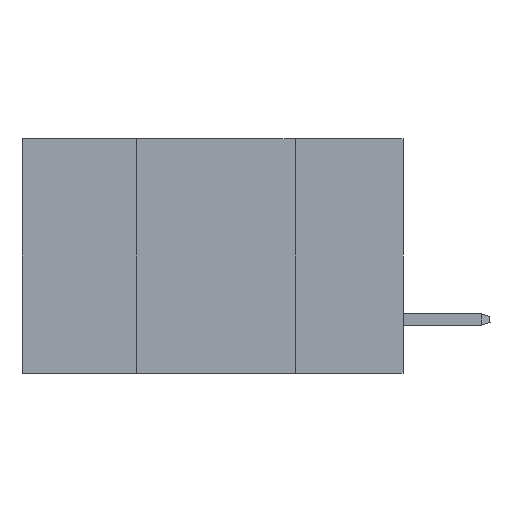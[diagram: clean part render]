
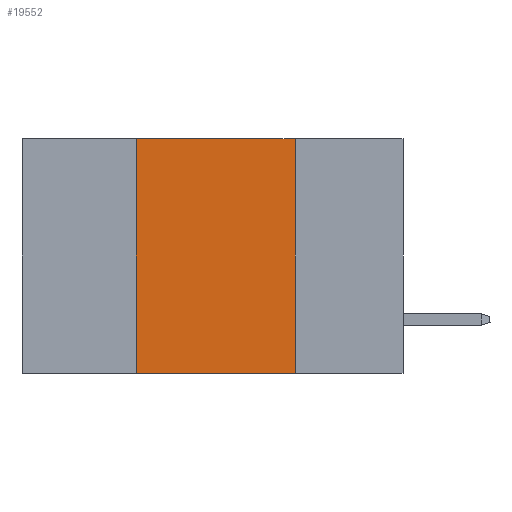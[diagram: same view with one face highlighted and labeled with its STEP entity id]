
A CAD part, left-side view. The second image highlights one B-rep face of the part: STEP entity #19552.
In plain terms, the highlighted planar face has unit normal (-1, 0, 0).
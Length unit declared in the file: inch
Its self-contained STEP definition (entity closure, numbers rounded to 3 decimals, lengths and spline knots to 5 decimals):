
#427 = EDGE_CURVE ( 'NONE', #15564, #19002, #16780, .T. ) ;
#1391 = VECTOR ( 'NONE', #14733, 39.37008 ) ;
#1635 = LINE ( 'NONE', #17211, #10752 ) ;
#1637 = VERTEX_POINT ( 'NONE', #1924 ) ;
#1669 = CARTESIAN_POINT ( 'NONE',  ( 0., 0.17, 0. ) ) ;
#1924 = CARTESIAN_POINT ( 'NONE',  ( 0., 0.42, 0. ) ) ;
#2098 = ORIENTED_EDGE ( 'NONE', *, *, #19156, .T. ) ;
#2625 = DIRECTION ( 'NONE',  ( 0., -1., 0. ) ) ;
#5854 = PLANE ( 'NONE',  #12537 ) ;
#6512 = DIRECTION ( 'NONE',  ( 0., -1., 0. ) ) ;
#8509 = CARTESIAN_POINT ( 'NONE',  ( 0., 0.6, 0. ) ) ;
#8519 = CARTESIAN_POINT ( 'NONE',  ( 0., 0.17, 0. ) ) ;
#8749 = EDGE_CURVE ( 'NONE', #1637, #15564, #1635, .T. ) ;
#9951 = VECTOR ( 'NONE', #2625, 39.37008 ) ;
#10146 = VECTOR ( 'NONE', #12488, 39.37008 ) ;
#10369 = FACE_OUTER_BOUND ( 'NONE', #18367, .T. ) ;
#10752 = VECTOR ( 'NONE', #6512, 39.37008 ) ;
#11020 = CARTESIAN_POINT ( 'NONE',  ( 0., 0.17, -0.37 ) ) ;
#12104 = CARTESIAN_POINT ( 'NONE',  ( 0., 0.6, -0.37 ) ) ;
#12220 = EDGE_CURVE ( 'NONE', #17898, #1637, #13999, .T. ) ;
#12488 = DIRECTION ( 'NONE',  ( 0., 0., 1. ) ) ;
#12537 = AXIS2_PLACEMENT_3D ( 'NONE', #8509, #17982, #19608 ) ;
#13020 = CARTESIAN_POINT ( 'NONE',  ( 0., 0.42, -0.37 ) ) ;
#13384 = ORIENTED_EDGE ( 'NONE', *, *, #8749, .F. ) ;
#13775 = ORIENTED_EDGE ( 'NONE', *, *, #427, .F. ) ;
#13999 = LINE ( 'NONE', #18886, #10146 ) ;
#14733 = DIRECTION ( 'NONE',  ( 0., 0., -1. ) ) ;
#15564 = VERTEX_POINT ( 'NONE', #1669 ) ;
#16287 = ORIENTED_EDGE ( 'NONE', *, *, #12220, .F. ) ;
#16385 = LINE ( 'NONE', #12104, #9951 ) ;
#16780 = LINE ( 'NONE', #8519, #1391 ) ;
#17211 = CARTESIAN_POINT ( 'NONE',  ( 0., 0.6, 0. ) ) ;
#17898 = VERTEX_POINT ( 'NONE', #13020 ) ;
#17982 = DIRECTION ( 'NONE',  ( 1., 0., 0. ) ) ;
#18367 = EDGE_LOOP ( 'NONE', ( #13775, #13384, #16287, #2098 ) ) ;
#18886 = CARTESIAN_POINT ( 'NONE',  ( 0., 0.42, 0. ) ) ;
#19002 = VERTEX_POINT ( 'NONE', #11020 ) ;
#19156 = EDGE_CURVE ( 'NONE', #17898, #19002, #16385, .T. ) ;
#19552 = ADVANCED_FACE ( 'NONE', ( #10369 ), #5854, .F. ) ;
#19608 = DIRECTION ( 'NONE',  ( 0., 0., -1. ) ) ;
